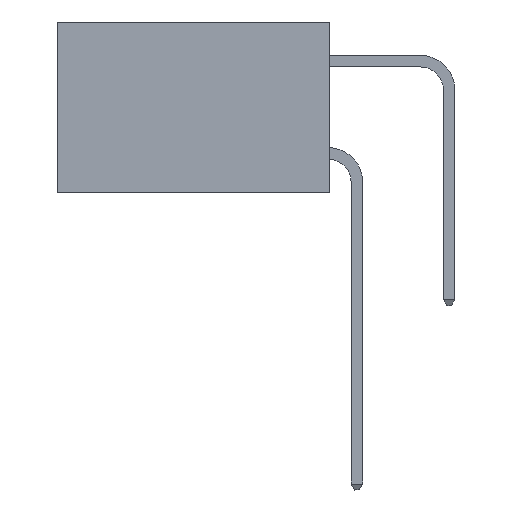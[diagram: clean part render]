
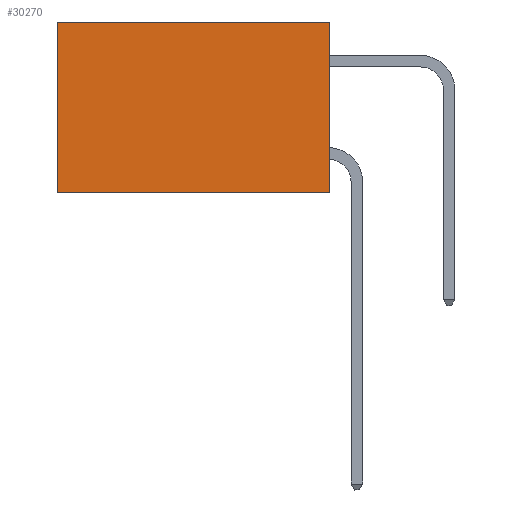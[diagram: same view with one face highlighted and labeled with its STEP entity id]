
A CAD part, left-side view. The second image highlights one B-rep face of the part: STEP entity #30270.
In plain terms, the highlighted planar face has unit normal (-1, 0, 0).
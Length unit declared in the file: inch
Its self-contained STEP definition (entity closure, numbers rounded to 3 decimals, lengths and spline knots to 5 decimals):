
#773 = EDGE_CURVE ( 'NONE', #3206, #30279, #13302, .T. ) ;
#852 = EDGE_CURVE ( 'NONE', #3206, #19737, #23750, .T. ) ;
#1979 = DIRECTION ( 'NONE',  ( 0., 1., 0. ) ) ;
#3206 = VERTEX_POINT ( 'NONE', #7581 ) ;
#4110 = VECTOR ( 'NONE', #1979, 39.37008 ) ;
#4655 = AXIS2_PLACEMENT_3D ( 'NONE', #12342, #31834, #15145 ) ;
#5140 = CARTESIAN_POINT ( 'NONE',  ( 0.277, 0., 0. ) ) ;
#7482 = ORIENTED_EDGE ( 'NONE', *, *, #773, .T. ) ;
#7581 = CARTESIAN_POINT ( 'NONE',  ( 0.277, 0., 0. ) ) ;
#7620 = ORIENTED_EDGE ( 'NONE', *, *, #35443, .F. ) ;
#7850 = LINE ( 'NONE', #26344, #22691 ) ;
#8038 = VERTEX_POINT ( 'NONE', #32605 ) ;
#9102 = ORIENTED_EDGE ( 'NONE', *, *, #852, .F. ) ;
#9245 = EDGE_CURVE ( 'NONE', #30279, #8038, #7850, .T. ) ;
#9615 = DIRECTION ( 'NONE',  ( 0., 0., -1. ) ) ;
#10484 = LINE ( 'NONE', #30998, #16167 ) ;
#12342 = CARTESIAN_POINT ( 'NONE',  ( 0.277, 0., -0.37 ) ) ;
#13302 = LINE ( 'NONE', #5140, #4110 ) ;
#14999 = CARTESIAN_POINT ( 'NONE',  ( 0.277, 0., -0.37 ) ) ;
#15145 = DIRECTION ( 'NONE',  ( 0., 0., -1. ) ) ;
#16167 = VECTOR ( 'NONE', #33768, 39.37008 ) ;
#16367 = VECTOR ( 'NONE', #35578, 39.37008 ) ;
#17093 = EDGE_LOOP ( 'NONE', ( #26000, #7620, #9102, #7482 ) ) ;
#17948 = CARTESIAN_POINT ( 'NONE',  ( 0.277, 0.59, 0. ) ) ;
#19737 = VERTEX_POINT ( 'NONE', #28070 ) ;
#22691 = VECTOR ( 'NONE', #9615, 39.37008 ) ;
#23750 = LINE ( 'NONE', #14999, #16367 ) ;
#26000 = ORIENTED_EDGE ( 'NONE', *, *, #9245, .T. ) ;
#26344 = CARTESIAN_POINT ( 'NONE',  ( 0.277, 0.59, -0.37 ) ) ;
#28070 = CARTESIAN_POINT ( 'NONE',  ( 0.277, 0., -0.37 ) ) ;
#29051 = PLANE ( 'NONE',  #4655 ) ;
#30270 = ADVANCED_FACE ( 'NONE', ( #31788 ), #29051, .F. ) ;
#30279 = VERTEX_POINT ( 'NONE', #17948 ) ;
#30998 = CARTESIAN_POINT ( 'NONE',  ( 0.277, 0., -0.37 ) ) ;
#31788 = FACE_OUTER_BOUND ( 'NONE', #17093, .T. ) ;
#31834 = DIRECTION ( 'NONE',  ( 1., 0., 0. ) ) ;
#32605 = CARTESIAN_POINT ( 'NONE',  ( 0.277, 0.59, -0.37 ) ) ;
#33768 = DIRECTION ( 'NONE',  ( 0., 1., 0. ) ) ;
#35443 = EDGE_CURVE ( 'NONE', #19737, #8038, #10484, .T. ) ;
#35578 = DIRECTION ( 'NONE',  ( 0., 0., -1. ) ) ;
